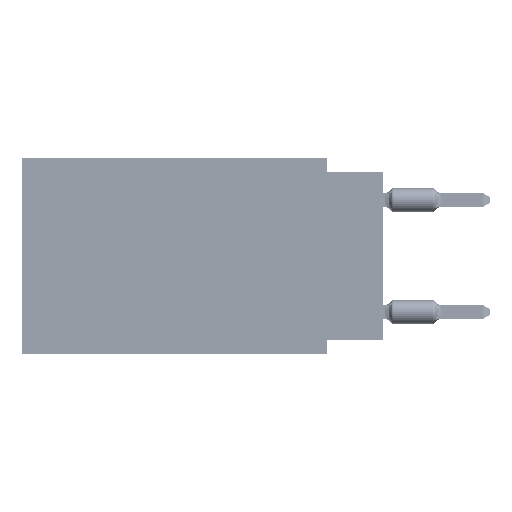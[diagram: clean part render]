
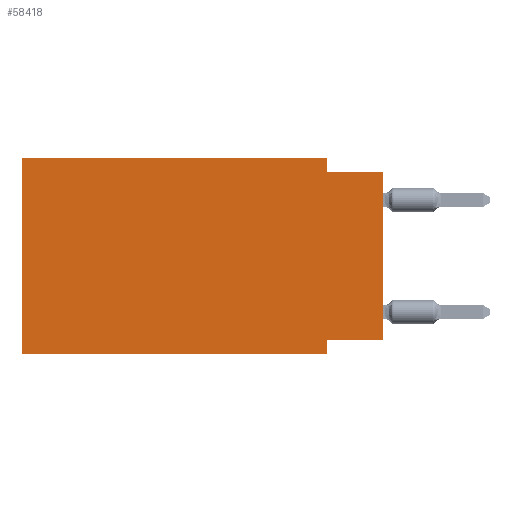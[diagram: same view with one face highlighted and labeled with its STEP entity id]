
A CAD part, left-side view. The second image highlights one B-rep face of the part: STEP entity #58418.
In plain terms, the highlighted planar face has unit normal (-1, 0, 0).
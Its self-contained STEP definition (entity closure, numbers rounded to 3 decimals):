
#865 = PLANE ( 'NONE',  #3655 ) ;
#2158 = CARTESIAN_POINT ( 'NONE',  ( 0., 2.54, -8.255 ) ) ;
#3655 = AXIS2_PLACEMENT_3D ( 'NONE', #28719, #63415, #51606 ) ;
#3709 = CARTESIAN_POINT ( 'NONE',  ( 0., 2.54, -8.89 ) ) ;
#7824 = VERTEX_POINT ( 'NONE', #2158 ) ;
#7926 = CARTESIAN_POINT ( 'NONE',  ( 0., 16.383, -8.89 ) ) ;
#8684 = DIRECTION ( 'NONE',  ( 0., -1., 0. ) ) ;
#8775 = LINE ( 'NONE', #27057, #63507 ) ;
#9320 = EDGE_CURVE ( 'NONE', #47695, #37941, #9493, .T. ) ;
#9493 = LINE ( 'NONE', #22059, #43817 ) ;
#12625 = VECTOR ( 'NONE', #23472, 1000. ) ;
#13793 = DIRECTION ( 'NONE',  ( 0., 0., 1. ) ) ;
#15832 = LINE ( 'NONE', #72997, #33907 ) ;
#16759 = EDGE_LOOP ( 'NONE', ( #57616, #22924, #47067, #63560, #49472, #64378, #33867, #55298 ) ) ;
#16816 = VECTOR ( 'NONE', #20872, 1000. ) ;
#18943 = EDGE_CURVE ( 'NONE', #47695, #7824, #15832, .T. ) ;
#20135 = CARTESIAN_POINT ( 'NONE',  ( 0., 16.383, 0. ) ) ;
#20487 = DIRECTION ( 'NONE',  ( 0., 0., -1. ) ) ;
#20824 = EDGE_CURVE ( 'NONE', #45949, #34920, #48484, .T. ) ;
#20872 = DIRECTION ( 'NONE',  ( 0., -1., 0. ) ) ;
#21445 = CARTESIAN_POINT ( 'NONE',  ( 0., 16.383, -8.89 ) ) ;
#22059 = CARTESIAN_POINT ( 'NONE',  ( 0., 0., 0. ) ) ;
#22440 = EDGE_CURVE ( 'NONE', #34920, #42962, #8775, .T. ) ;
#22450 = VECTOR ( 'NONE', #8684, 1000. ) ;
#22924 = ORIENTED_EDGE ( 'NONE', *, *, #34905, .F. ) ;
#23472 = DIRECTION ( 'NONE',  ( 0., 0., -1. ) ) ;
#25824 = LINE ( 'NONE', #7926, #22450 ) ;
#27057 = CARTESIAN_POINT ( 'NONE',  ( 0., 16.383, 0. ) ) ;
#28719 = CARTESIAN_POINT ( 'NONE',  ( 0., 16.383, 0. ) ) ;
#30146 = CARTESIAN_POINT ( 'NONE',  ( 0., 0., -8.255 ) ) ;
#33867 = ORIENTED_EDGE ( 'NONE', *, *, #57424, .F. ) ;
#33907 = VECTOR ( 'NONE', #62339, 1000. ) ;
#34905 = EDGE_CURVE ( 'NONE', #66112, #37941, #54834, .T. ) ;
#34920 = VERTEX_POINT ( 'NONE', #20135 ) ;
#37941 = VERTEX_POINT ( 'NONE', #51674 ) ;
#41272 = VECTOR ( 'NONE', #20487, 1000. ) ;
#41767 = CARTESIAN_POINT ( 'NONE',  ( 0., 2.54, 0. ) ) ;
#42962 = VERTEX_POINT ( 'NONE', #53206 ) ;
#43817 = VECTOR ( 'NONE', #56767, 1000. ) ;
#44147 = CARTESIAN_POINT ( 'NONE',  ( 0., 2.54, -0.635 ) ) ;
#44788 = VERTEX_POINT ( 'NONE', #45831 ) ;
#44988 = DIRECTION ( 'NONE',  ( 0., -1., 0. ) ) ;
#45831 = CARTESIAN_POINT ( 'NONE',  ( 0., 2.54, -8.89 ) ) ;
#45949 = VERTEX_POINT ( 'NONE', #21445 ) ;
#47067 = ORIENTED_EDGE ( 'NONE', *, *, #51420, .F. ) ;
#47498 = LINE ( 'NONE', #41767, #12625 ) ;
#47517 = VECTOR ( 'NONE', #13793, 1000. ) ;
#47695 = VERTEX_POINT ( 'NONE', #30146 ) ;
#48190 = EDGE_CURVE ( 'NONE', #45949, #44788, #25824, .T. ) ;
#48484 = LINE ( 'NONE', #71709, #47517 ) ;
#49472 = ORIENTED_EDGE ( 'NONE', *, *, #20824, .F. ) ;
#51420 = EDGE_CURVE ( 'NONE', #42962, #66112, #47498, .T. ) ;
#51606 = DIRECTION ( 'NONE',  ( 0., 0., -1. ) ) ;
#51674 = CARTESIAN_POINT ( 'NONE',  ( 0., 0., -0.635 ) ) ;
#53206 = CARTESIAN_POINT ( 'NONE',  ( 0., 2.54, 0. ) ) ;
#54834 = LINE ( 'NONE', #66259, #16816 ) ;
#55298 = ORIENTED_EDGE ( 'NONE', *, *, #18943, .F. ) ;
#56767 = DIRECTION ( 'NONE',  ( 0., 0., 1. ) ) ;
#57424 = EDGE_CURVE ( 'NONE', #7824, #44788, #66991, .T. ) ;
#57616 = ORIENTED_EDGE ( 'NONE', *, *, #9320, .T. ) ;
#58418 = ADVANCED_FACE ( 'NONE', ( #64531 ), #865, .F. ) ;
#62339 = DIRECTION ( 'NONE',  ( 0., 1., 0. ) ) ;
#63415 = DIRECTION ( 'NONE',  ( 1., 0., 0. ) ) ;
#63507 = VECTOR ( 'NONE', #44988, 1000. ) ;
#63560 = ORIENTED_EDGE ( 'NONE', *, *, #22440, .F. ) ;
#64378 = ORIENTED_EDGE ( 'NONE', *, *, #48190, .T. ) ;
#64531 = FACE_OUTER_BOUND ( 'NONE', #16759, .T. ) ;
#66112 = VERTEX_POINT ( 'NONE', #44147 ) ;
#66259 = CARTESIAN_POINT ( 'NONE',  ( 0., 0., -0.635 ) ) ;
#66991 = LINE ( 'NONE', #3709, #41272 ) ;
#71709 = CARTESIAN_POINT ( 'NONE',  ( 0., 16.383, 0. ) ) ;
#72997 = CARTESIAN_POINT ( 'NONE',  ( 0., 0., -8.255 ) ) ;
